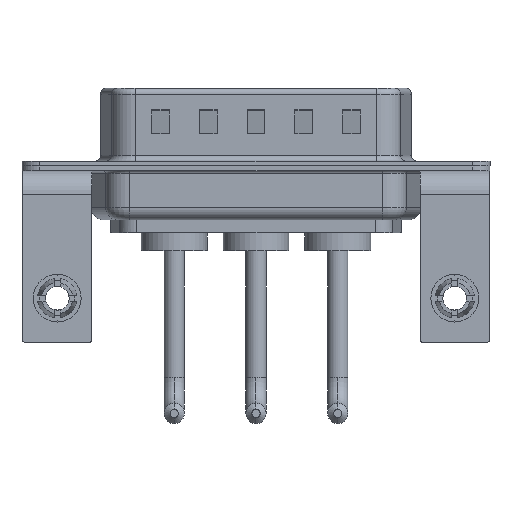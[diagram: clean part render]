
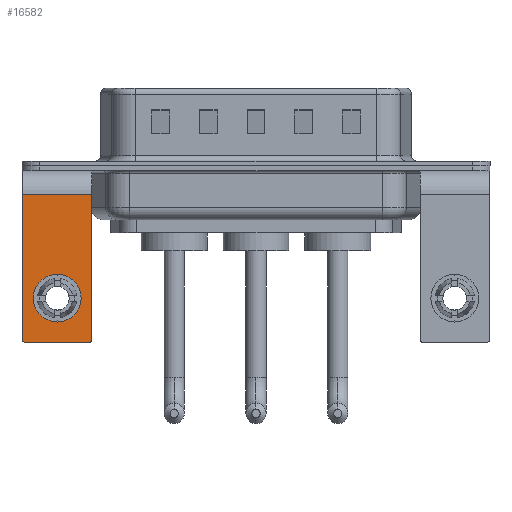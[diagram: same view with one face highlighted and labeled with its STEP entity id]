
A CAD part, front view. The second image highlights one B-rep face of the part: STEP entity #16582.
In plain terms, the highlighted planar face has unit normal (0, -1, 0).
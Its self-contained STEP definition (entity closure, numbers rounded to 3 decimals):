
#54 = PLANE ( 'NONE',  #10504 ) ;
#123 = CARTESIAN_POINT ( 'NONE',  ( 0., -6.25, -11.07 ) ) ;
#264 = VERTEX_POINT ( 'NONE', #10275 ) ;
#429 = DIRECTION ( 'NONE',  ( -1., 0., 0. ) ) ;
#473 = ORIENTED_EDGE ( 'NONE', *, *, #6865, .T. ) ;
#621 = EDGE_CURVE ( 'NONE', #10557, #264, #12911, .T. ) ;
#1351 = CARTESIAN_POINT ( 'NONE',  ( -2.65, -6.25, -14.8 ) ) ;
#1431 = FACE_OUTER_BOUND ( 'NONE', #16050, .T. ) ;
#1640 = ORIENTED_EDGE ( 'NONE', *, *, #621, .T. ) ;
#1656 = VERTEX_POINT ( 'NONE', #1679 ) ;
#1679 = CARTESIAN_POINT ( 'NONE',  ( 2.9, -6.25, -14.55 ) ) ;
#1987 = EDGE_CURVE ( 'NONE', #7075, #1656, #2509, .T. ) ;
#2333 = CARTESIAN_POINT ( 'NONE',  ( 2.9, -6.25, -2.4 ) ) ;
#2509 = LINE ( 'NONE', #6653, #6674 ) ;
#2704 = AXIS2_PLACEMENT_3D ( 'NONE', #123, #5748, #16999 ) ;
#3030 = ORIENTED_EDGE ( 'NONE', *, *, #16215, .T. ) ;
#3132 = VECTOR ( 'NONE', #9947, 1000. ) ;
#3206 = VERTEX_POINT ( 'NONE', #8992 ) ;
#3591 = CIRCLE ( 'NONE', #15081, 0.25 ) ;
#3827 = ORIENTED_EDGE ( 'NONE', *, *, #13178, .F. ) ;
#4373 = CARTESIAN_POINT ( 'NONE',  ( 2.9, -6.25, -2.4 ) ) ;
#4520 = VERTEX_POINT ( 'NONE', #11942 ) ;
#4985 = AXIS2_PLACEMENT_3D ( 'NONE', #18225, #13943, #17172 ) ;
#5527 = LINE ( 'NONE', #5710, #3132 ) ;
#5710 = CARTESIAN_POINT ( 'NONE',  ( -2.9, -6.25, -2.4 ) ) ;
#5748 = DIRECTION ( 'NONE',  ( 0., 1., 0. ) ) ;
#6006 = VECTOR ( 'NONE', #7414, 1000. ) ;
#6524 = CARTESIAN_POINT ( 'NONE',  ( 0., -6.25, -13.07 ) ) ;
#6653 = CARTESIAN_POINT ( 'NONE',  ( 2.9, -6.25, -2.4 ) ) ;
#6674 = VECTOR ( 'NONE', #18104, 1000. ) ;
#6865 = EDGE_CURVE ( 'NONE', #264, #10557, #10352, .T. ) ;
#7075 = VERTEX_POINT ( 'NONE', #2333 ) ;
#7238 = ORIENTED_EDGE ( 'NONE', *, *, #10907, .T. ) ;
#7414 = DIRECTION ( 'NONE',  ( -1., 0., 0. ) ) ;
#7777 = VERTEX_POINT ( 'NONE', #1351 ) ;
#7810 = VECTOR ( 'NONE', #429, 1000. ) ;
#8347 = EDGE_LOOP ( 'NONE', ( #1640, #473 ) ) ;
#8404 = LINE ( 'NONE', #9853, #7810 ) ;
#8427 = CARTESIAN_POINT ( 'NONE',  ( 2.65, -6.25, -14.55 ) ) ;
#8735 = CIRCLE ( 'NONE', #11074, 0.25 ) ;
#8957 = CARTESIAN_POINT ( 'NONE',  ( -2.9, -6.25, -14.55 ) ) ;
#8992 = CARTESIAN_POINT ( 'NONE',  ( 2.65, -6.25, -14.8 ) ) ;
#9064 = CARTESIAN_POINT ( 'NONE',  ( 2.9, -6.25, -14.8 ) ) ;
#9106 = EDGE_CURVE ( 'NONE', #4520, #14978, #5527, .T. ) ;
#9853 = CARTESIAN_POINT ( 'NONE',  ( 2.9, -6.25, -2.4 ) ) ;
#9947 = DIRECTION ( 'NONE',  ( 0., 0., -1. ) ) ;
#9997 = DIRECTION ( 'NONE',  ( 0., 1., 0. ) ) ;
#10098 = CARTESIAN_POINT ( 'NONE',  ( -2.65, -6.25, -14.55 ) ) ;
#10275 = CARTESIAN_POINT ( 'NONE',  ( 0., -6.25, -9.07 ) ) ;
#10352 = CIRCLE ( 'NONE', #2704, 2. ) ;
#10504 = AXIS2_PLACEMENT_3D ( 'NONE', #4373, #9997, #15622 ) ;
#10557 = VERTEX_POINT ( 'NONE', #6524 ) ;
#10907 = EDGE_CURVE ( 'NONE', #14978, #7777, #3591, .T. ) ;
#11074 = AXIS2_PLACEMENT_3D ( 'NONE', #8427, #14212, #17168 ) ;
#11672 = DIRECTION ( 'NONE',  ( 0., 0., 1. ) ) ;
#11942 = CARTESIAN_POINT ( 'NONE',  ( -2.9, -6.25, -2.4 ) ) ;
#12516 = ORIENTED_EDGE ( 'NONE', *, *, #9106, .T. ) ;
#12911 = CIRCLE ( 'NONE', #4985, 2. ) ;
#13178 = EDGE_CURVE ( 'NONE', #3206, #7777, #13311, .T. ) ;
#13191 = ORIENTED_EDGE ( 'NONE', *, *, #15178, .T. ) ;
#13311 = LINE ( 'NONE', #9064, #6006 ) ;
#13943 = DIRECTION ( 'NONE',  ( 0., 1., 0. ) ) ;
#14212 = DIRECTION ( 'NONE',  ( 0., -1., 0. ) ) ;
#14620 = DIRECTION ( 'NONE',  ( 0., -1., 0. ) ) ;
#14978 = VERTEX_POINT ( 'NONE', #8957 ) ;
#15081 = AXIS2_PLACEMENT_3D ( 'NONE', #10098, #14620, #11672 ) ;
#15178 = EDGE_CURVE ( 'NONE', #7075, #4520, #8404, .T. ) ;
#15622 = DIRECTION ( 'NONE',  ( 0., 0., 1. ) ) ;
#16050 = EDGE_LOOP ( 'NONE', ( #12516, #7238, #3827, #3030, #17720, #13191 ) ) ;
#16215 = EDGE_CURVE ( 'NONE', #3206, #1656, #8735, .T. ) ;
#16582 = ADVANCED_FACE ( 'NONE', ( #17015, #1431 ), #54, .F. ) ;
#16999 = DIRECTION ( 'NONE',  ( 0., 0., 1. ) ) ;
#17015 = FACE_BOUND ( 'NONE', #8347, .T. ) ;
#17168 = DIRECTION ( 'NONE',  ( 0., 0., 1. ) ) ;
#17172 = DIRECTION ( 'NONE',  ( 0., 0., 1. ) ) ;
#17720 = ORIENTED_EDGE ( 'NONE', *, *, #1987, .F. ) ;
#18104 = DIRECTION ( 'NONE',  ( 0., 0., -1. ) ) ;
#18225 = CARTESIAN_POINT ( 'NONE',  ( 0., -6.25, -11.07 ) ) ;
